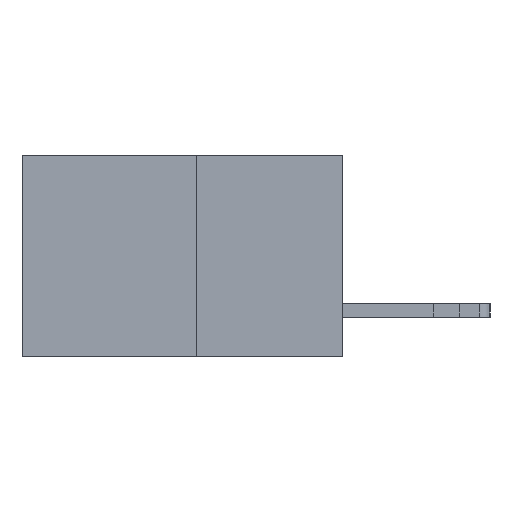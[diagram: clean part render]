
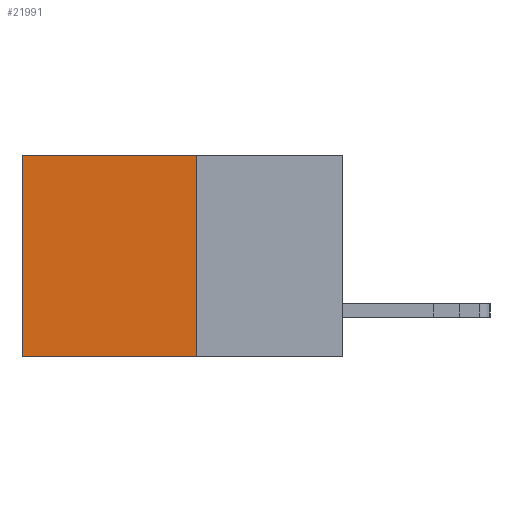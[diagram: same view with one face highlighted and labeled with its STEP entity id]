
A CAD part, left-side view. The second image highlights one B-rep face of the part: STEP entity #21991.
In plain terms, the highlighted planar face has unit normal (-1, 0, 0).
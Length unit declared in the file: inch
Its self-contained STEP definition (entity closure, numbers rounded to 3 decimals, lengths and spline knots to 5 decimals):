
#771 = VECTOR ( 'NONE', #14815, 39.37008 ) ;
#917 = DIRECTION ( 'NONE',  ( 0., 1., 0. ) ) ;
#992 = VERTEX_POINT ( 'NONE', #21936 ) ;
#1161 = FACE_OUTER_BOUND ( 'NONE', #19300, .T. ) ;
#1379 = CARTESIAN_POINT ( 'NONE',  ( 0.277, 0.59, -0.37 ) ) ;
#1634 = DIRECTION ( 'NONE',  ( 0., 0., -1. ) ) ;
#2325 = EDGE_CURVE ( 'NONE', #14238, #8945, #18476, .T. ) ;
#2625 = CARTESIAN_POINT ( 'NONE',  ( 0.277, 0.27, -0.37 ) ) ;
#2919 = VERTEX_POINT ( 'NONE', #18930 ) ;
#3766 = ORIENTED_EDGE ( 'NONE', *, *, #2325, .F. ) ;
#3793 = LINE ( 'NONE', #5254, #15015 ) ;
#4208 = CARTESIAN_POINT ( 'NONE',  ( 0.277, 0.59, -0.37 ) ) ;
#5254 = CARTESIAN_POINT ( 'NONE',  ( 0.277, 0.27, -0.37 ) ) ;
#8945 = VERTEX_POINT ( 'NONE', #1379 ) ;
#10917 = EDGE_CURVE ( 'NONE', #992, #2919, #11250, .T. ) ;
#11250 = LINE ( 'NONE', #23981, #16153 ) ;
#11609 = VECTOR ( 'NONE', #917, 39.37008 ) ;
#11630 = DIRECTION ( 'NONE',  ( 0., 1., 0. ) ) ;
#12073 = LINE ( 'NONE', #4208, #771 ) ;
#14238 = VERTEX_POINT ( 'NONE', #25619 ) ;
#14318 = DIRECTION ( 'NONE',  ( 1., 0., 0. ) ) ;
#14815 = DIRECTION ( 'NONE',  ( 0., 0., -1. ) ) ;
#15015 = VECTOR ( 'NONE', #19967, 39.37008 ) ;
#15082 = AXIS2_PLACEMENT_3D ( 'NONE', #26642, #14318, #1634 ) ;
#16153 = VECTOR ( 'NONE', #11630, 39.37008 ) ;
#16204 = EDGE_CURVE ( 'NONE', #992, #14238, #3793, .T. ) ;
#17099 = EDGE_CURVE ( 'NONE', #2919, #8945, #12073, .T. ) ;
#18367 = ORIENTED_EDGE ( 'NONE', *, *, #17099, .T. ) ;
#18476 = LINE ( 'NONE', #2625, #11609 ) ;
#18930 = CARTESIAN_POINT ( 'NONE',  ( 0.277, 0.59, 0. ) ) ;
#19300 = EDGE_LOOP ( 'NONE', ( #18367, #3766, #23802, #26175 ) ) ;
#19967 = DIRECTION ( 'NONE',  ( 0., 0., -1. ) ) ;
#21936 = CARTESIAN_POINT ( 'NONE',  ( 0.277, 0.27, 0. ) ) ;
#21991 = ADVANCED_FACE ( 'NONE', ( #1161 ), #22582, .F. ) ;
#22582 = PLANE ( 'NONE',  #15082 ) ;
#23802 = ORIENTED_EDGE ( 'NONE', *, *, #16204, .F. ) ;
#23981 = CARTESIAN_POINT ( 'NONE',  ( 0.277, 0.27, 0. ) ) ;
#25619 = CARTESIAN_POINT ( 'NONE',  ( 0.277, 0.27, -0.37 ) ) ;
#26175 = ORIENTED_EDGE ( 'NONE', *, *, #10917, .T. ) ;
#26642 = CARTESIAN_POINT ( 'NONE',  ( 0.277, 0.27, -0.37 ) ) ;
